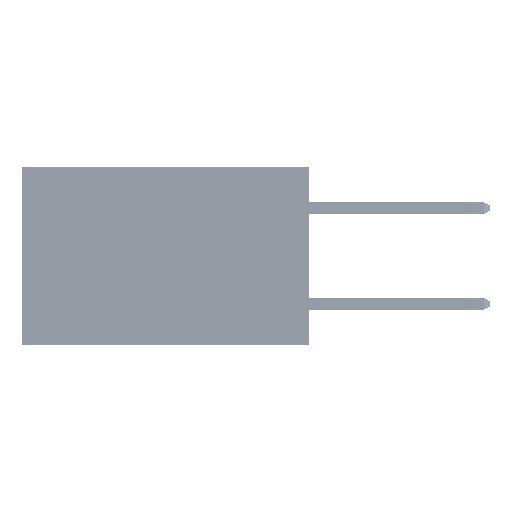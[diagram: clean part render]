
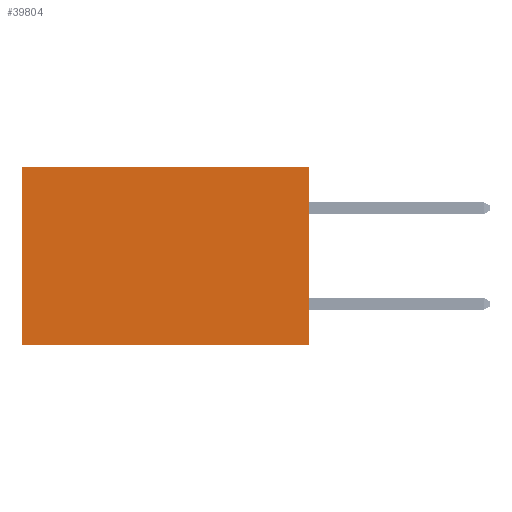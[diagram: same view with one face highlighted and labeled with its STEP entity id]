
A CAD part, left-side view. The second image highlights one B-rep face of the part: STEP entity #39804.
In plain terms, the highlighted planar face has unit normal (-1, 0, 0).
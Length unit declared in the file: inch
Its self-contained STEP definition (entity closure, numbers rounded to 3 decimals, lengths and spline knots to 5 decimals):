
#1069 = DIRECTION ( 'NONE',  ( 0., 1., 0. ) ) ;
#1412 = CARTESIAN_POINT ( 'NONE',  ( 0.2875, 0.6, 0. ) ) ;
#3969 = VECTOR ( 'NONE', #36250, 39.37008 ) ;
#6028 = ORIENTED_EDGE ( 'NONE', *, *, #26090, .F. ) ;
#6293 = EDGE_CURVE ( 'NONE', #8835, #29299, #19895, .T. ) ;
#8358 = EDGE_CURVE ( 'NONE', #29299, #25764, #14260, .T. ) ;
#8835 = VERTEX_POINT ( 'NONE', #49882 ) ;
#9198 = CARTESIAN_POINT ( 'NONE',  ( 0.2875, 0., -0.37 ) ) ;
#10266 = FACE_OUTER_BOUND ( 'NONE', #44540, .T. ) ;
#10381 = DIRECTION ( 'NONE',  ( 1., 0., 0. ) ) ;
#12958 = DIRECTION ( 'NONE',  ( 0., 1., 0. ) ) ;
#14260 = LINE ( 'NONE', #1412, #3969 ) ;
#18518 = PLANE ( 'NONE',  #24696 ) ;
#19392 = CARTESIAN_POINT ( 'NONE',  ( 0.2875, 0.6, -0.37 ) ) ;
#19895 = LINE ( 'NONE', #35400, #30299 ) ;
#20721 = VECTOR ( 'NONE', #12958, 39.37008 ) ;
#20836 = ORIENTED_EDGE ( 'NONE', *, *, #32124, .F. ) ;
#23790 = LINE ( 'NONE', #9198, #20721 ) ;
#24415 = CARTESIAN_POINT ( 'NONE',  ( 0.2875, 0., 0. ) ) ;
#24696 = AXIS2_PLACEMENT_3D ( 'NONE', #29437, #10381, #29597 ) ;
#25764 = VERTEX_POINT ( 'NONE', #19392 ) ;
#26090 = EDGE_CURVE ( 'NONE', #29380, #25764, #23790, .T. ) ;
#26289 = VECTOR ( 'NONE', #47994, 39.37008 ) ;
#29299 = VERTEX_POINT ( 'NONE', #43752 ) ;
#29380 = VERTEX_POINT ( 'NONE', #35748 ) ;
#29437 = CARTESIAN_POINT ( 'NONE',  ( 0.2875, 0., 0. ) ) ;
#29597 = DIRECTION ( 'NONE',  ( 0., 0., -1. ) ) ;
#30299 = VECTOR ( 'NONE', #1069, 39.37008 ) ;
#32124 = EDGE_CURVE ( 'NONE', #8835, #29380, #44541, .T. ) ;
#35400 = CARTESIAN_POINT ( 'NONE',  ( 0.2875, 0., 0. ) ) ;
#35748 = CARTESIAN_POINT ( 'NONE',  ( 0.2875, 0., -0.37 ) ) ;
#36250 = DIRECTION ( 'NONE',  ( 0., 0., -1. ) ) ;
#37005 = ORIENTED_EDGE ( 'NONE', *, *, #6293, .T. ) ;
#39804 = ADVANCED_FACE ( 'NONE', ( #10266 ), #18518, .F. ) ;
#43752 = CARTESIAN_POINT ( 'NONE',  ( 0.2875, 0.6, 0. ) ) ;
#44540 = EDGE_LOOP ( 'NONE', ( #47515, #6028, #20836, #37005 ) ) ;
#44541 = LINE ( 'NONE', #24415, #26289 ) ;
#47515 = ORIENTED_EDGE ( 'NONE', *, *, #8358, .T. ) ;
#47994 = DIRECTION ( 'NONE',  ( 0., 0., -1. ) ) ;
#49882 = CARTESIAN_POINT ( 'NONE',  ( 0.2875, 0., 0. ) ) ;
